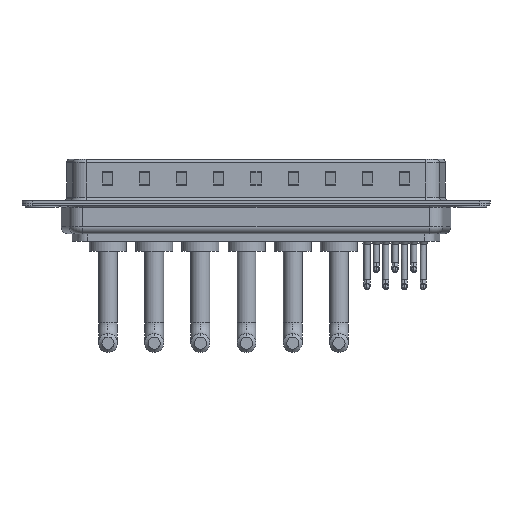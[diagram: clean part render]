
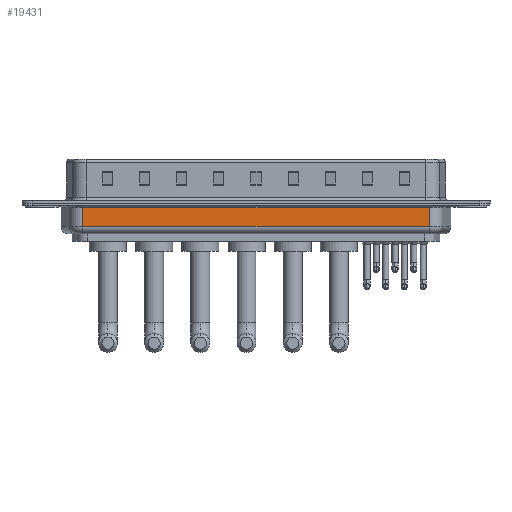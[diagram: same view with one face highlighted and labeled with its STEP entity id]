
A CAD part, front view. The second image highlights one B-rep face of the part: STEP entity #19431.
In plain terms, the highlighted planar face has unit normal (0, -1, 0).
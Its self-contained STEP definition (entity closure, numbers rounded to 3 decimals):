
#697 = EDGE_CURVE ( 'NONE', #4044, #15039, #1330, .T. ) ;
#792 = VECTOR ( 'NONE', #22559, 1000. ) ;
#915 = PLANE ( 'NONE',  #14956 ) ;
#1330 = LINE ( 'NONE', #4901, #792 ) ;
#1639 = CARTESIAN_POINT ( 'NONE',  ( 57.469, -5.35, -4.5 ) ) ;
#1802 = LINE ( 'NONE', #9006, #16076 ) ;
#4044 = VERTEX_POINT ( 'NONE', #12299 ) ;
#4219 = VERTEX_POINT ( 'NONE', #5738 ) ;
#4464 = FACE_OUTER_BOUND ( 'NONE', #11193, .T. ) ;
#4781 = EDGE_CURVE ( 'NONE', #4044, #7718, #9629, .T. ) ;
#4901 = CARTESIAN_POINT ( 'NONE',  ( 6.031, -5.35, -3.5 ) ) ;
#4977 = DIRECTION ( 'NONE',  ( 0., 0., 1. ) ) ;
#5116 = VECTOR ( 'NONE', #4977, 1000. ) ;
#5738 = CARTESIAN_POINT ( 'NONE',  ( 57.469, -5.35, -0.65 ) ) ;
#6069 = DIRECTION ( 'NONE',  ( 0., 1., 0. ) ) ;
#6419 = CARTESIAN_POINT ( 'NONE',  ( 6.031, -5.35, -4.5 ) ) ;
#6436 = CARTESIAN_POINT ( 'NONE',  ( 6.031, -5.35, -4.5 ) ) ;
#7718 = VERTEX_POINT ( 'NONE', #20206 ) ;
#8624 = LINE ( 'NONE', #1639, #5116 ) ;
#9006 = CARTESIAN_POINT ( 'NONE',  ( 6.031, -5.35, -0.65 ) ) ;
#9411 = ORIENTED_EDGE ( 'NONE', *, *, #21891, .T. ) ;
#9629 = LINE ( 'NONE', #6436, #13238 ) ;
#9742 = DIRECTION ( 'NONE',  ( 0., 0., 1. ) ) ;
#11193 = EDGE_LOOP ( 'NONE', ( #22630, #21857, #14099, #9411 ) ) ;
#11580 = DIRECTION ( 'NONE',  ( -1., 0., 0. ) ) ;
#12299 = CARTESIAN_POINT ( 'NONE',  ( 6.031, -5.35, -3.5 ) ) ;
#13238 = VECTOR ( 'NONE', #9742, 1000. ) ;
#14099 = ORIENTED_EDGE ( 'NONE', *, *, #22118, .T. ) ;
#14956 = AXIS2_PLACEMENT_3D ( 'NONE', #6419, #6069, #11580 ) ;
#15039 = VERTEX_POINT ( 'NONE', #18176 ) ;
#16076 = VECTOR ( 'NONE', #21287, 1000. ) ;
#18176 = CARTESIAN_POINT ( 'NONE',  ( 57.469, -5.35, -3.5 ) ) ;
#19431 = ADVANCED_FACE ( 'NONE', ( #4464 ), #915, .F. ) ;
#20206 = CARTESIAN_POINT ( 'NONE',  ( 6.031, -5.35, -0.65 ) ) ;
#21287 = DIRECTION ( 'NONE',  ( -1., 0., 0. ) ) ;
#21857 = ORIENTED_EDGE ( 'NONE', *, *, #697, .T. ) ;
#21891 = EDGE_CURVE ( 'NONE', #4219, #7718, #1802, .T. ) ;
#22118 = EDGE_CURVE ( 'NONE', #15039, #4219, #8624, .T. ) ;
#22559 = DIRECTION ( 'NONE',  ( 1., 0., 0. ) ) ;
#22630 = ORIENTED_EDGE ( 'NONE', *, *, #4781, .F. ) ;
